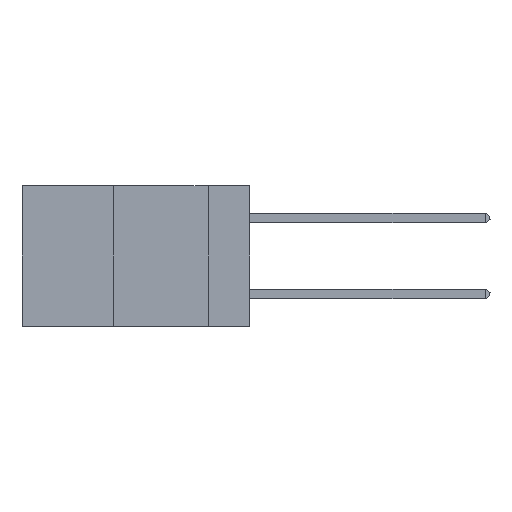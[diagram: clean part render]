
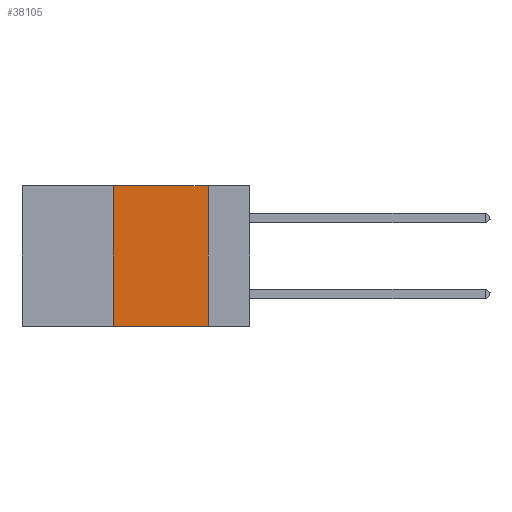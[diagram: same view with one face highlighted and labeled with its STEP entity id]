
A CAD part, left-side view. The second image highlights one B-rep face of the part: STEP entity #38105.
In plain terms, the highlighted planar face has unit normal (-1, 0, 0).
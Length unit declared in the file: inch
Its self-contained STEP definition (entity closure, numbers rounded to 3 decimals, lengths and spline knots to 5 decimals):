
#474 = ORIENTED_EDGE ( 'NONE', *, *, #39462, .T. ) ;
#575 = CARTESIAN_POINT ( 'NONE',  ( 0., 0.11, 0. ) ) ;
#3087 = VERTEX_POINT ( 'NONE', #575 ) ;
#6320 = ORIENTED_EDGE ( 'NONE', *, *, #18405, .F. ) ;
#6710 = VECTOR ( 'NONE', #7799, 39.37008 ) ;
#6824 = CARTESIAN_POINT ( 'NONE',  ( 0., 0.11, -0.37 ) ) ;
#7532 = VERTEX_POINT ( 'NONE', #32383 ) ;
#7572 = VECTOR ( 'NONE', #9226, 39.37008 ) ;
#7671 = VERTEX_POINT ( 'NONE', #33568 ) ;
#7799 = DIRECTION ( 'NONE',  ( 0., 0., 1. ) ) ;
#8366 = DIRECTION ( 'NONE',  ( 0., -1., 0. ) ) ;
#9226 = DIRECTION ( 'NONE',  ( 0., 0., -1. ) ) ;
#9528 = VECTOR ( 'NONE', #31302, 39.37008 ) ;
#9616 = AXIS2_PLACEMENT_3D ( 'NONE', #19683, #10554, #31820 ) ;
#10554 = DIRECTION ( 'NONE',  ( 1., 0., 0. ) ) ;
#11827 = EDGE_CURVE ( 'NONE', #3087, #21095, #15806, .T. ) ;
#15806 = LINE ( 'NONE', #36453, #7572 ) ;
#16426 = ORIENTED_EDGE ( 'NONE', *, *, #19601, .F. ) ;
#17711 = LINE ( 'NONE', #19162, #9528 ) ;
#17765 = LINE ( 'NONE', #26720, #32895 ) ;
#18405 = EDGE_CURVE ( 'NONE', #7671, #7532, #37166, .T. ) ;
#19162 = CARTESIAN_POINT ( 'NONE',  ( 0., 0.6, 0. ) ) ;
#19523 = EDGE_LOOP ( 'NONE', ( #24735, #16426, #6320, #474 ) ) ;
#19601 = EDGE_CURVE ( 'NONE', #7532, #3087, #17711, .T. ) ;
#19683 = CARTESIAN_POINT ( 'NONE',  ( 0., 0.6, 0. ) ) ;
#21095 = VERTEX_POINT ( 'NONE', #6824 ) ;
#23085 = CARTESIAN_POINT ( 'NONE',  ( 0., 0.36, 0. ) ) ;
#24735 = ORIENTED_EDGE ( 'NONE', *, *, #11827, .F. ) ;
#25803 = PLANE ( 'NONE',  #9616 ) ;
#26720 = CARTESIAN_POINT ( 'NONE',  ( 0., 0.6, -0.37 ) ) ;
#31302 = DIRECTION ( 'NONE',  ( 0., -1., 0. ) ) ;
#31820 = DIRECTION ( 'NONE',  ( 0., 0., -1. ) ) ;
#32383 = CARTESIAN_POINT ( 'NONE',  ( 0., 0.36, 0. ) ) ;
#32895 = VECTOR ( 'NONE', #8366, 39.37008 ) ;
#33568 = CARTESIAN_POINT ( 'NONE',  ( 0., 0.36, -0.37 ) ) ;
#36453 = CARTESIAN_POINT ( 'NONE',  ( 0., 0.11, 0. ) ) ;
#36767 = FACE_OUTER_BOUND ( 'NONE', #19523, .T. ) ;
#37166 = LINE ( 'NONE', #23085, #6710 ) ;
#38105 = ADVANCED_FACE ( 'NONE', ( #36767 ), #25803, .F. ) ;
#39462 = EDGE_CURVE ( 'NONE', #7671, #21095, #17765, .T. ) ;
